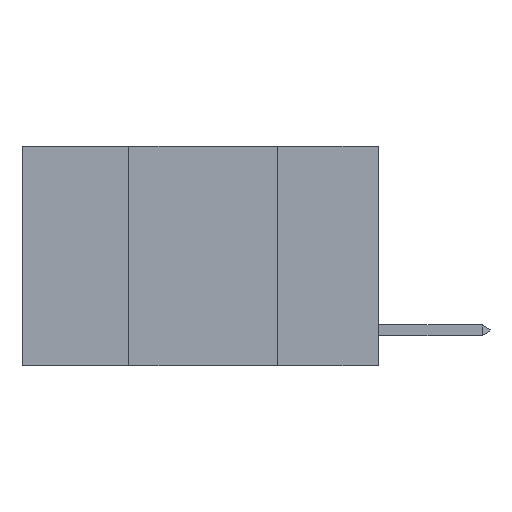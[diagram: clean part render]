
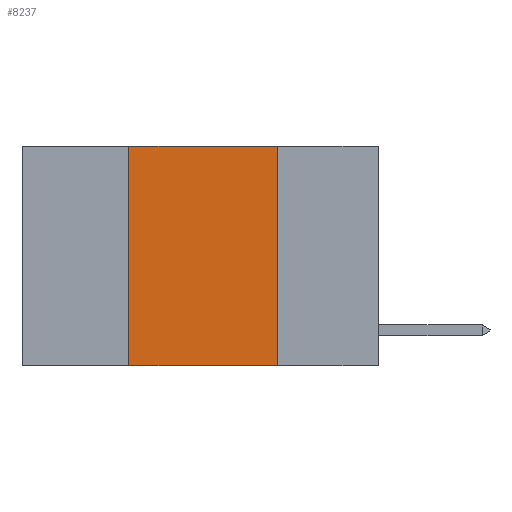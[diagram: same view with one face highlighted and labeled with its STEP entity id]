
A CAD part, left-side view. The second image highlights one B-rep face of the part: STEP entity #8237.
In plain terms, the highlighted planar face has unit normal (-1, 0, 0).
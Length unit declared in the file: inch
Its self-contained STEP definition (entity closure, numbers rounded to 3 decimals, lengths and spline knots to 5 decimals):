
#117 = VECTOR ( 'NONE', #11051, 39.37008 ) ;
#942 = VECTOR ( 'NONE', #23687, 39.37008 ) ;
#2009 = EDGE_CURVE ( 'NONE', #24546, #22209, #21822, .T. ) ;
#3220 = DIRECTION ( 'NONE',  ( 1., 0., 0. ) ) ;
#5173 = EDGE_CURVE ( 'NONE', #12182, #7321, #12352, .T. ) ;
#7321 = VERTEX_POINT ( 'NONE', #19190 ) ;
#7501 = CARTESIAN_POINT ( 'NONE',  ( 0., 0.6, 0. ) ) ;
#8022 = EDGE_CURVE ( 'NONE', #12182, #24546, #11565, .T. ) ;
#8237 = ADVANCED_FACE ( 'NONE', ( #16792 ), #24419, .F. ) ;
#8331 = AXIS2_PLACEMENT_3D ( 'NONE', #7501, #3220, #18146 ) ;
#9011 = CARTESIAN_POINT ( 'NONE',  ( 0., 0.17, 0. ) ) ;
#9581 = VECTOR ( 'NONE', #17582, 39.37008 ) ;
#11051 = DIRECTION ( 'NONE',  ( 0., 0., 1. ) ) ;
#11565 = LINE ( 'NONE', #25807, #117 ) ;
#12182 = VERTEX_POINT ( 'NONE', #22990 ) ;
#12352 = LINE ( 'NONE', #21585, #942 ) ;
#13996 = ORIENTED_EDGE ( 'NONE', *, *, #19356, .F. ) ;
#14649 = CARTESIAN_POINT ( 'NONE',  ( 0., 0.42, 0. ) ) ;
#14786 = ORIENTED_EDGE ( 'NONE', *, *, #2009, .F. ) ;
#15097 = ORIENTED_EDGE ( 'NONE', *, *, #8022, .F. ) ;
#15437 = CARTESIAN_POINT ( 'NONE',  ( 0., 0.17, 0. ) ) ;
#15894 = ORIENTED_EDGE ( 'NONE', *, *, #5173, .T. ) ;
#16792 = FACE_OUTER_BOUND ( 'NONE', #22314, .T. ) ;
#17582 = DIRECTION ( 'NONE',  ( 0., 0., -1. ) ) ;
#17961 = CARTESIAN_POINT ( 'NONE',  ( 0., 0.6, 0. ) ) ;
#18146 = DIRECTION ( 'NONE',  ( 0., 0., -1. ) ) ;
#19190 = CARTESIAN_POINT ( 'NONE',  ( 0., 0.17, -0.37 ) ) ;
#19356 = EDGE_CURVE ( 'NONE', #22209, #7321, #27080, .T. ) ;
#21137 = VECTOR ( 'NONE', #24334, 39.37008 ) ;
#21585 = CARTESIAN_POINT ( 'NONE',  ( 0., 0.6, -0.37 ) ) ;
#21822 = LINE ( 'NONE', #17961, #21137 ) ;
#22209 = VERTEX_POINT ( 'NONE', #9011 ) ;
#22314 = EDGE_LOOP ( 'NONE', ( #13996, #14786, #15097, #15894 ) ) ;
#22990 = CARTESIAN_POINT ( 'NONE',  ( 0., 0.42, -0.37 ) ) ;
#23687 = DIRECTION ( 'NONE',  ( 0., -1., 0. ) ) ;
#24334 = DIRECTION ( 'NONE',  ( 0., -1., 0. ) ) ;
#24419 = PLANE ( 'NONE',  #8331 ) ;
#24546 = VERTEX_POINT ( 'NONE', #14649 ) ;
#25807 = CARTESIAN_POINT ( 'NONE',  ( 0., 0.42, 0. ) ) ;
#27080 = LINE ( 'NONE', #15437, #9581 ) ;
